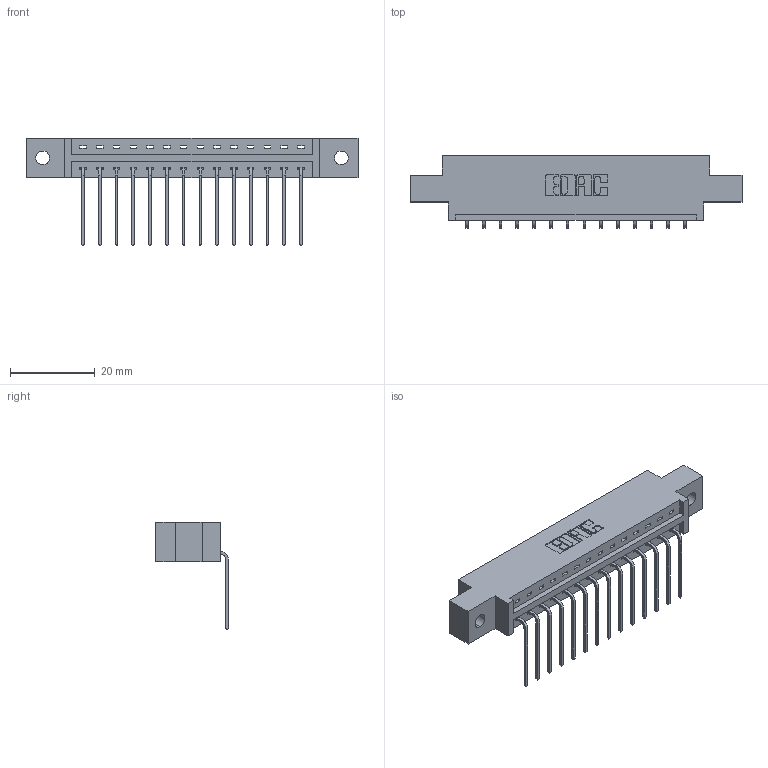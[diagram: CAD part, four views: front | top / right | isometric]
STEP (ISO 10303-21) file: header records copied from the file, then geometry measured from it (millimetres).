
FILE_DESCRIPTION (( 'STEP AP203' ), '1' );
FILE_NAME ('387-014-559-602.STEP', '2018-09-11T06:28:45', ( '' ), ( '' ), 'SwSTEP 2.0', 'SolidWorks 2016', '' );
FILE_SCHEMA (( 'CONFIG_CONTROL_DESIGN' ));
Length unit declared in the file: inch
Products named in the file (3): 337 Part_0.170 Offset - 0.128 Dia; 345-292-001_558 559 Tail - 1; 387-014-559-602
Assembly tree (15 placements, depth 2):
  387-014-559-602
    337 Part_0.170 Offset - 0.128 Dia
    345-292-001_558 559 Tail - 1  x14
Bounding box: 78.49 x 17.09 x 25.53 mm (x, y, z)
Volume: 7699.4 mm3; surface area: 7913.9 mm2
Topology: 15 solids, 15 shells, 1014 faces, 3039 edges, 2006 vertices
Faces by surface type: plane 746, cylinder 268
Entity records: 14247 total; most frequent: CARTESIAN_POINT 2488, ORIENTED_EDGE 2438, DIRECTION 2151, EDGE_CURVE 1219, VECTOR 1091, LINE 1091, VERTEX_POINT 810, AXIS2_PLACEMENT_3D 530
